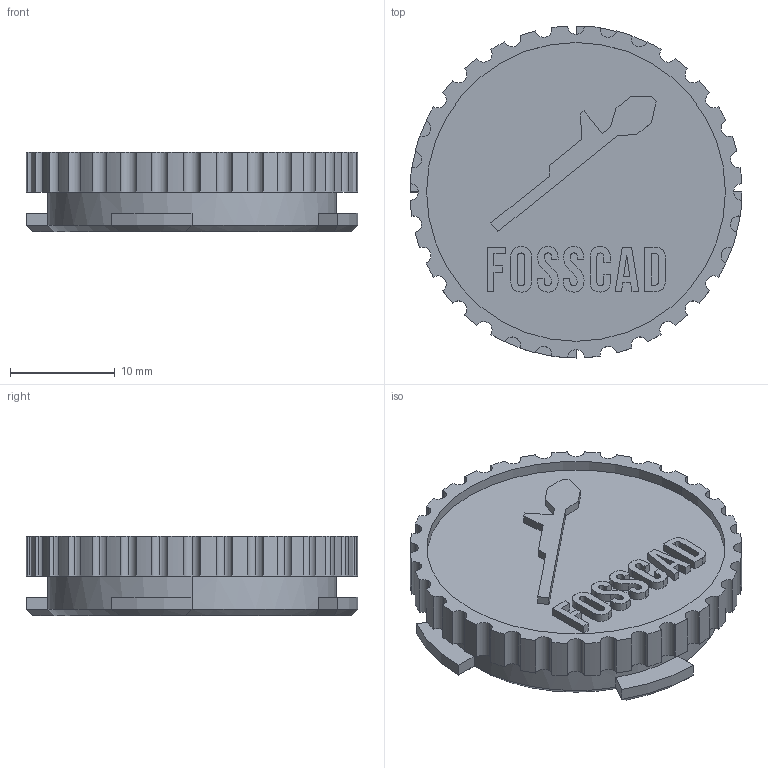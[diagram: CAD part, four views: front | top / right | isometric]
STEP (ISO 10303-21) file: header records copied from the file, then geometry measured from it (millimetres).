
FILE_DESCRIPTION (( 'STEP AP203' ), '1' );
FILE_NAME ('AF-HF-TK-PRT-008-STEP_FOSSCAD.STEP', '2020-12-04T15:25:51', ( '' ), ( '' ), 'SwSTEP 2.0', 'SolidWorks 2018', '' );
FILE_SCHEMA (( 'CONFIG_CONTROL_DESIGN' ));
Length unit declared in the file: inch
Products named in the file (1): AF-HF-TK-PRT-008-STEP_FOSSCAD
Bounding box: 31.75 x 31.75 x 7.62 mm (x, y, z)
Volume: 3717.4 mm3; surface area: 2768.7 mm2
Topology: 1 solids, 1 shells, 253 faces, 687 edges, 450 vertices
Faces by surface type: plane 105, cylinder 89, bspline 44, cone 13, sphere 2
Entity records: 10263 total; most frequent: CARTESIAN_POINT 3947, ORIENTED_EDGE 1374, DIRECTION 1202, EDGE_CURVE 687, VERTEX_POINT 450, AXIS2_PLACEMENT_3D 409, VECTOR 384, LINE 384
